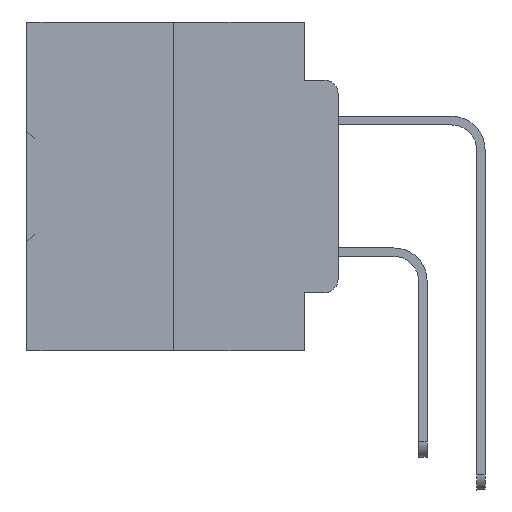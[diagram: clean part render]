
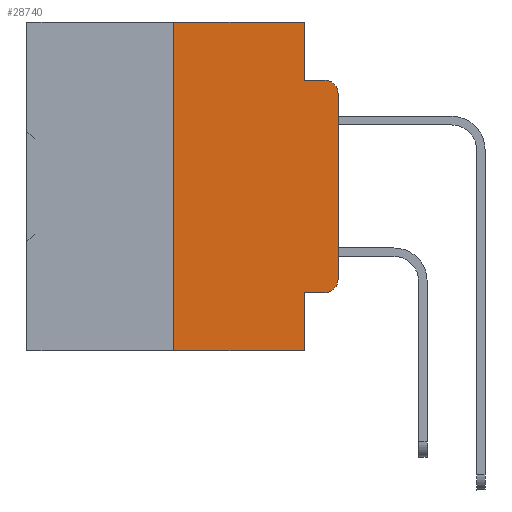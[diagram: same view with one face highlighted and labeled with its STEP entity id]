
A CAD part, left-side view. The second image highlights one B-rep face of the part: STEP entity #28740.
In plain terms, the highlighted planar face has unit normal (-1, 0, 0).
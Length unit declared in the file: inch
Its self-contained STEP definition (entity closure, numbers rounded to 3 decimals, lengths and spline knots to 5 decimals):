
#393 = DIRECTION ( 'NONE',  ( 0., 0., -1. ) ) ;
#1146 = AXIS2_PLACEMENT_3D ( 'NONE', #25104, #28389, #393 ) ;
#1545 = EDGE_LOOP ( 'NONE', ( #31896, #29944, #27611, #37252, #25156, #1900, #16416, #17959, #16042, #14362 ) ) ;
#1652 = EDGE_CURVE ( 'NONE', #16203, #7435, #17703, .T. ) ;
#1900 = ORIENTED_EDGE ( 'NONE', *, *, #21173, .F. ) ;
#1949 = DIRECTION ( 'NONE',  ( -1., 0., 0. ) ) ;
#2310 = LINE ( 'NONE', #33553, #35225 ) ;
#2527 = DIRECTION ( 'NONE',  ( 0., 0., -1. ) ) ;
#2924 = DIRECTION ( 'NONE',  ( 0., 0., -1. ) ) ;
#3752 = AXIS2_PLACEMENT_3D ( 'NONE', #34506, #19557, #6534 ) ;
#5301 = VERTEX_POINT ( 'NONE', #20324 ) ;
#5596 = CARTESIAN_POINT ( 'NONE',  ( 0., 0.051, 0. ) ) ;
#6047 = VERTEX_POINT ( 'NONE', #36006 ) ;
#6534 = DIRECTION ( 'NONE',  ( 0., 0., -1. ) ) ;
#6719 = CARTESIAN_POINT ( 'NONE',  ( 0., 0.051, -0.0885 ) ) ;
#6724 = FACE_OUTER_BOUND ( 'NONE', #1545, .T. ) ;
#7112 = DIRECTION ( 'NONE',  ( 0., 0., 1. ) ) ;
#7435 = VERTEX_POINT ( 'NONE', #31088 ) ;
#7769 = CARTESIAN_POINT ( 'NONE',  ( 0., 0.051, -0.5 ) ) ;
#8242 = VERTEX_POINT ( 'NONE', #20086 ) ;
#9088 = CARTESIAN_POINT ( 'NONE',  ( 0., 0.02, -0.4115 ) ) ;
#10347 = VECTOR ( 'NONE', #22087, 39.37008 ) ;
#14236 = VERTEX_POINT ( 'NONE', #9088 ) ;
#14362 = ORIENTED_EDGE ( 'NONE', *, *, #28027, .T. ) ;
#14639 = CARTESIAN_POINT ( 'NONE',  ( 0., 0.051, -0.0885 ) ) ;
#16042 = ORIENTED_EDGE ( 'NONE', *, *, #19247, .T. ) ;
#16203 = VERTEX_POINT ( 'NONE', #6719 ) ;
#16416 = ORIENTED_EDGE ( 'NONE', *, *, #19985, .T. ) ;
#16688 = CIRCLE ( 'NONE', #21902, 0.02 ) ;
#17077 = DIRECTION ( 'NONE',  ( 0., 0., 1. ) ) ;
#17659 = VECTOR ( 'NONE', #2924, 39.37008 ) ;
#17703 = LINE ( 'NONE', #14639, #24928 ) ;
#17887 = EDGE_CURVE ( 'NONE', #6047, #7435, #35689, .T. ) ;
#17959 = ORIENTED_EDGE ( 'NONE', *, *, #34411, .F. ) ;
#18133 = VERTEX_POINT ( 'NONE', #24043 ) ;
#19247 = EDGE_CURVE ( 'NONE', #22830, #14236, #37828, .T. ) ;
#19557 = DIRECTION ( 'NONE',  ( 1., 0., 0. ) ) ;
#19593 = CARTESIAN_POINT ( 'NONE',  ( 0., 0.25, -0.5 ) ) ;
#19985 = EDGE_CURVE ( 'NONE', #25024, #39621, #24415, .T. ) ;
#20086 = CARTESIAN_POINT ( 'NONE',  ( 0., 0.25, 0. ) ) ;
#20206 = LINE ( 'NONE', #32668, #35571 ) ;
#20324 = CARTESIAN_POINT ( 'NONE',  ( 0., 0.051, 0. ) ) ;
#20357 = EDGE_CURVE ( 'NONE', #5301, #16203, #2310, .T. ) ;
#21173 = EDGE_CURVE ( 'NONE', #25024, #8242, #25084, .T. ) ;
#21902 = AXIS2_PLACEMENT_3D ( 'NONE', #23983, #1949, #24195 ) ;
#21934 = CARTESIAN_POINT ( 'NONE',  ( 0., 0.473, -0.5 ) ) ;
#22087 = DIRECTION ( 'NONE',  ( 0., -1., 0. ) ) ;
#22418 = PLANE ( 'NONE',  #3752 ) ;
#22830 = VERTEX_POINT ( 'NONE', #27935 ) ;
#23003 = VECTOR ( 'NONE', #17077, 39.37008 ) ;
#23983 = CARTESIAN_POINT ( 'NONE',  ( 0., 0.02, -0.3915 ) ) ;
#24043 = CARTESIAN_POINT ( 'NONE',  ( 0., 0., -0.3915 ) ) ;
#24195 = DIRECTION ( 'NONE',  ( 0., 0., -1. ) ) ;
#24415 = LINE ( 'NONE', #21934, #25433 ) ;
#24928 = VECTOR ( 'NONE', #33046, 39.37008 ) ;
#25024 = VERTEX_POINT ( 'NONE', #19593 ) ;
#25084 = LINE ( 'NONE', #35093, #30030 ) ;
#25104 = CARTESIAN_POINT ( 'NONE',  ( 0., 0.02, -0.1085 ) ) ;
#25156 = ORIENTED_EDGE ( 'NONE', *, *, #39664, .F. ) ;
#25433 = VECTOR ( 'NONE', #28897, 39.37008 ) ;
#26090 = CARTESIAN_POINT ( 'NONE',  ( 0., 0., 0. ) ) ;
#27611 = ORIENTED_EDGE ( 'NONE', *, *, #1652, .F. ) ;
#27854 = LINE ( 'NONE', #5596, #17659 ) ;
#27935 = CARTESIAN_POINT ( 'NONE',  ( 0., 0.051, -0.4115 ) ) ;
#28027 = EDGE_CURVE ( 'NONE', #14236, #18133, #16688, .T. ) ;
#28389 = DIRECTION ( 'NONE',  ( -1., 0., 0. ) ) ;
#28447 = CARTESIAN_POINT ( 'NONE',  ( 0., 0.051, -0.4115 ) ) ;
#28740 = ADVANCED_FACE ( 'NONE', ( #6724 ), #22418, .F. ) ;
#28897 = DIRECTION ( 'NONE',  ( 0., -1., 0. ) ) ;
#29159 = LINE ( 'NONE', #26090, #23003 ) ;
#29944 = ORIENTED_EDGE ( 'NONE', *, *, #17887, .T. ) ;
#30030 = VECTOR ( 'NONE', #7112, 39.37008 ) ;
#31088 = CARTESIAN_POINT ( 'NONE',  ( 0., 0.02, -0.0885 ) ) ;
#31896 = ORIENTED_EDGE ( 'NONE', *, *, #35553, .T. ) ;
#32668 = CARTESIAN_POINT ( 'NONE',  ( 0., 0.473, 0. ) ) ;
#33046 = DIRECTION ( 'NONE',  ( 0., -1., 0. ) ) ;
#33553 = CARTESIAN_POINT ( 'NONE',  ( 0., 0.051, 0. ) ) ;
#34411 = EDGE_CURVE ( 'NONE', #22830, #39621, #27854, .T. ) ;
#34506 = CARTESIAN_POINT ( 'NONE',  ( 0., 0.473, 0. ) ) ;
#35093 = CARTESIAN_POINT ( 'NONE',  ( 0., 0.25, 0. ) ) ;
#35225 = VECTOR ( 'NONE', #2527, 39.37008 ) ;
#35553 = EDGE_CURVE ( 'NONE', #18133, #6047, #29159, .T. ) ;
#35571 = VECTOR ( 'NONE', #37995, 39.37008 ) ;
#35689 = CIRCLE ( 'NONE', #1146, 0.02 ) ;
#36006 = CARTESIAN_POINT ( 'NONE',  ( 0., 0., -0.1085 ) ) ;
#37252 = ORIENTED_EDGE ( 'NONE', *, *, #20357, .F. ) ;
#37828 = LINE ( 'NONE', #28447, #10347 ) ;
#37995 = DIRECTION ( 'NONE',  ( 0., -1., 0. ) ) ;
#39621 = VERTEX_POINT ( 'NONE', #7769 ) ;
#39664 = EDGE_CURVE ( 'NONE', #8242, #5301, #20206, .T. ) ;
